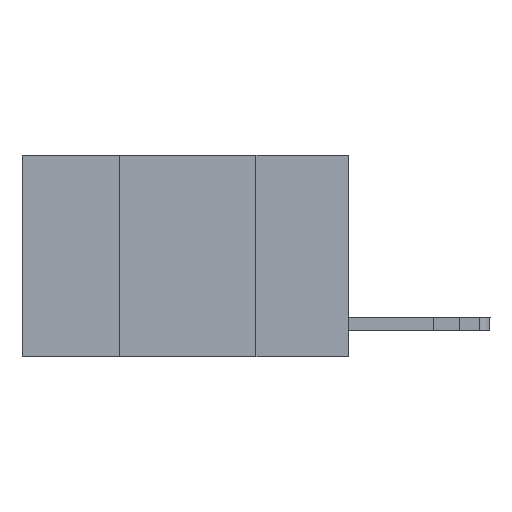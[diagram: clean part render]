
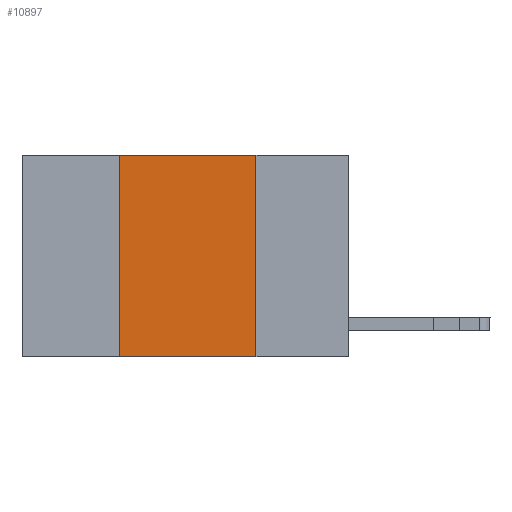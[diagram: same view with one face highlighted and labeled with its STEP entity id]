
A CAD part, left-side view. The second image highlights one B-rep face of the part: STEP entity #10897.
In plain terms, the highlighted planar face has unit normal (-1, 0, 0).
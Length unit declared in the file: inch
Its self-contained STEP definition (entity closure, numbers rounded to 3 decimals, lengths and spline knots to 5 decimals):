
#530 = CARTESIAN_POINT ( 'NONE',  ( 0., 0.42, 0. ) ) ;
#1366 = VECTOR ( 'NONE', #13664, 39.37008 ) ;
#1682 = CARTESIAN_POINT ( 'NONE',  ( 0., 0.17, 0. ) ) ;
#2864 = PLANE ( 'NONE',  #5155 ) ;
#3481 = CARTESIAN_POINT ( 'NONE',  ( 0., 0.17, 0. ) ) ;
#3721 = EDGE_CURVE ( 'NONE', #4132, #4017, #6645, .T. ) ;
#4017 = VERTEX_POINT ( 'NONE', #1682 ) ;
#4132 = VERTEX_POINT ( 'NONE', #530 ) ;
#4551 = CARTESIAN_POINT ( 'NONE',  ( 0., 0.17, -0.37 ) ) ;
#5024 = EDGE_CURVE ( 'NONE', #11738, #9396, #8175, .T. ) ;
#5155 = AXIS2_PLACEMENT_3D ( 'NONE', #13024, #13120, #14554 ) ;
#5392 = CARTESIAN_POINT ( 'NONE',  ( 0., 0.42, -0.37 ) ) ;
#6088 = DIRECTION ( 'NONE',  ( 0., -1., 0. ) ) ;
#6575 = ORIENTED_EDGE ( 'NONE', *, *, #15186, .F. ) ;
#6629 = LINE ( 'NONE', #12417, #1366 ) ;
#6645 = LINE ( 'NONE', #10823, #8718 ) ;
#8083 = CARTESIAN_POINT ( 'NONE',  ( 0., 0.6, -0.37 ) ) ;
#8146 = DIRECTION ( 'NONE',  ( 0., 0., -1. ) ) ;
#8175 = LINE ( 'NONE', #8083, #10208 ) ;
#8329 = VECTOR ( 'NONE', #8146, 39.37008 ) ;
#8718 = VECTOR ( 'NONE', #12342, 39.37008 ) ;
#9396 = VERTEX_POINT ( 'NONE', #4551 ) ;
#9544 = ORIENTED_EDGE ( 'NONE', *, *, #5024, .T. ) ;
#9850 = ORIENTED_EDGE ( 'NONE', *, *, #18172, .F. ) ;
#10208 = VECTOR ( 'NONE', #6088, 39.37008 ) ;
#10823 = CARTESIAN_POINT ( 'NONE',  ( 0., 0.6, 0. ) ) ;
#10897 = ADVANCED_FACE ( 'NONE', ( #17577 ), #2864, .F. ) ;
#11686 = EDGE_LOOP ( 'NONE', ( #9850, #16601, #6575, #9544 ) ) ;
#11738 = VERTEX_POINT ( 'NONE', #5392 ) ;
#12127 = LINE ( 'NONE', #3481, #8329 ) ;
#12342 = DIRECTION ( 'NONE',  ( 0., -1., 0. ) ) ;
#12417 = CARTESIAN_POINT ( 'NONE',  ( 0., 0.42, 0. ) ) ;
#13024 = CARTESIAN_POINT ( 'NONE',  ( 0., 0.6, 0. ) ) ;
#13120 = DIRECTION ( 'NONE',  ( 1., 0., 0. ) ) ;
#13664 = DIRECTION ( 'NONE',  ( 0., 0., 1. ) ) ;
#14554 = DIRECTION ( 'NONE',  ( 0., 0., -1. ) ) ;
#15186 = EDGE_CURVE ( 'NONE', #11738, #4132, #6629, .T. ) ;
#16601 = ORIENTED_EDGE ( 'NONE', *, *, #3721, .F. ) ;
#17577 = FACE_OUTER_BOUND ( 'NONE', #11686, .T. ) ;
#18172 = EDGE_CURVE ( 'NONE', #4017, #9396, #12127, .T. ) ;
